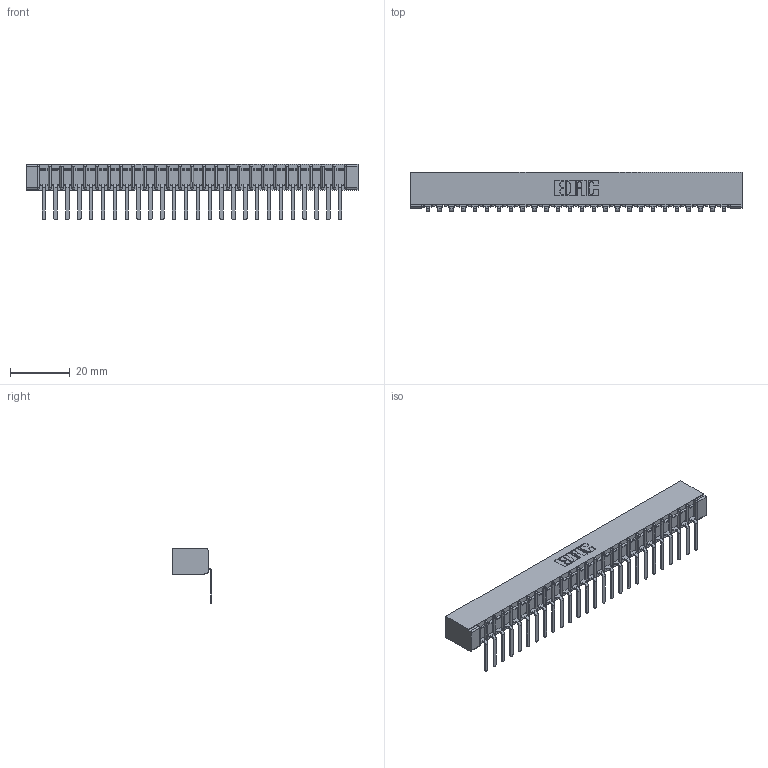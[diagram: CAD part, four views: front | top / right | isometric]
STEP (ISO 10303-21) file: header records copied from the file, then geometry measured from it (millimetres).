
FILE_DESCRIPTION (( 'STEP AP203' ), '1' );
FILE_NAME ('307-026-557-101.STEP', '2018-08-04T14:09:59', ( '' ), ( '' ), 'SwSTEP 2.0', 'SolidWorks 2016', '' );
FILE_SCHEMA (( 'CONFIG_CONTROL_DESIGN' ));
Length unit declared in the file: inch
Products named in the file (3): 307-290-002_557; 307-026-557-101; 307 Part_No Mounting Lugs
Assembly tree (27 placements, depth 2):
  307-026-557-101
    307 Part_No Mounting Lugs
    307-290-002_557  x26
Bounding box: 110.9 x 13.32 x 18.67 mm (x, y, z)
Volume: 7635.7 mm3; surface area: 15046.5 mm2
Topology: 27 solids, 27 shells, 2165 faces, 6643 edges, 4354 vertices
Faces by surface type: plane 1288, cylinder 823, sphere 54
Entity records: 24838 total; most frequent: CARTESIAN_POINT 4188, ORIENTED_EDGE 4178, DIRECTION 4075, EDGE_CURVE 2089, VECTOR 1593, LINE 1593, VERTEX_POINT 1354, AXIS2_PLACEMENT_3D 1241
